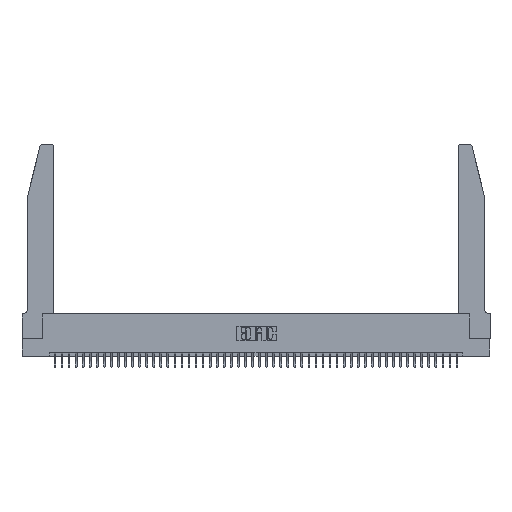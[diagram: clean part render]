
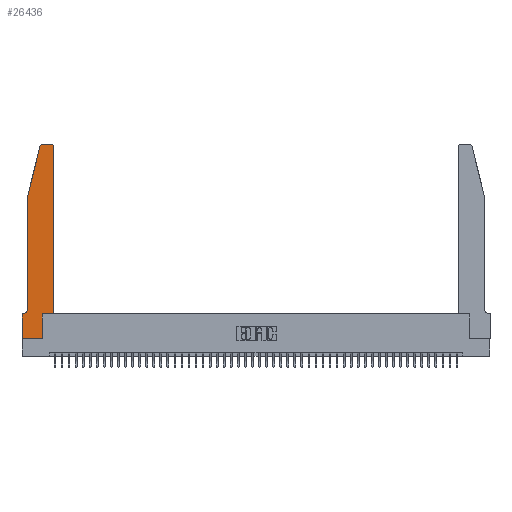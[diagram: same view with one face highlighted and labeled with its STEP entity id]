
A CAD part, top view. The second image highlights one B-rep face of the part: STEP entity #26436.
In plain terms, the highlighted planar face has unit normal (0, 0, 1).
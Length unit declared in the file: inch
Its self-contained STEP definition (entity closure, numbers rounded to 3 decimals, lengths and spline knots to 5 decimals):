
#658 = VERTEX_POINT ( 'NONE', #26307 ) ;
#1588 = VECTOR ( 'NONE', #24765, 39.37008 ) ;
#2399 = DIRECTION ( 'NONE',  ( -1., 0., 0. ) ) ;
#2454 = CARTESIAN_POINT ( 'NONE',  ( 0.0755, 0.42, 0.37 ) ) ;
#3434 = ORIENTED_EDGE ( 'NONE', *, *, #21208, .T. ) ;
#3478 = AXIS2_PLACEMENT_3D ( 'NONE', #16453, #45983, #41892 ) ;
#3490 = DIRECTION ( 'NONE',  ( 0., 0., 1. ) ) ;
#3765 = DIRECTION ( 'NONE',  ( -1., 0., 0. ) ) ;
#3785 = VERTEX_POINT ( 'NONE', #10804 ) ;
#3979 = CARTESIAN_POINT ( 'NONE',  ( 0.4205, 2.75, 0.37 ) ) ;
#4256 = CARTESIAN_POINT ( 'NONE',  ( 0., 0.35, 0.37 ) ) ;
#4416 = EDGE_CURVE ( 'NONE', #3785, #11045, #40281, .T. ) ;
#4452 = EDGE_CURVE ( 'NONE', #6735, #21793, #17524, .T. ) ;
#4508 = VECTOR ( 'NONE', #2399, 39.37008 ) ;
#4516 = VERTEX_POINT ( 'NONE', #4256 ) ;
#4940 = EDGE_CURVE ( 'NONE', #14509, #18523, #5757, .T. ) ;
#5757 = LINE ( 'NONE', #31956, #9851 ) ;
#5879 = CARTESIAN_POINT ( 'NONE',  ( 0.2865, 0.35, 0.37 ) ) ;
#6735 = VERTEX_POINT ( 'NONE', #46002 ) ;
#7153 = DIRECTION ( 'NONE',  ( 1., 0., 0. ) ) ;
#7306 = DIRECTION ( 'NONE',  ( 0., 1., 0. ) ) ;
#7971 = CARTESIAN_POINT ( 'NONE',  ( 0.2605, 2.75, 0.37 ) ) ;
#8220 = LINE ( 'NONE', #44546, #10585 ) ;
#8233 = ORIENTED_EDGE ( 'NONE', *, *, #4416, .T. ) ;
#8945 = VECTOR ( 'NONE', #47856, 39.37008 ) ;
#8959 = ORIENTED_EDGE ( 'NONE', *, *, #26096, .T. ) ;
#9250 = CARTESIAN_POINT ( 'NONE',  ( 0.4505, 2.72, 0.37 ) ) ;
#9505 = CARTESIAN_POINT ( 'NONE',  ( 0.2865, 0., 0.37 ) ) ;
#9851 = VECTOR ( 'NONE', #42897, 39.37008 ) ;
#10045 = CARTESIAN_POINT ( 'NONE',  ( 0.0755, 0.35, 0.37 ) ) ;
#10092 = CARTESIAN_POINT ( 'NONE',  ( 0., 0.35, 0.37 ) ) ;
#10585 = VECTOR ( 'NONE', #7306, 39.37008 ) ;
#10605 = CARTESIAN_POINT ( 'NONE',  ( 0.4505, 0.35, 0.37 ) ) ;
#10804 = CARTESIAN_POINT ( 'NONE',  ( 0.2865, 0.35, 0.37 ) ) ;
#11045 = VERTEX_POINT ( 'NONE', #23323 ) ;
#11275 = VERTEX_POINT ( 'NONE', #2454 ) ;
#13034 = PLANE ( 'NONE',  #36398 ) ;
#13481 = EDGE_CURVE ( 'NONE', #11045, #39683, #8220, .T. ) ;
#14509 = VERTEX_POINT ( 'NONE', #41894 ) ;
#14809 = FACE_OUTER_BOUND ( 'NONE', #20285, .T. ) ;
#14943 = ORIENTED_EDGE ( 'NONE', *, *, #48194, .T. ) ;
#15462 = EDGE_CURVE ( 'NONE', #39683, #21573, #30190, .T. ) ;
#15581 = DIRECTION ( 'NONE',  ( 1., 0., 0. ) ) ;
#15683 = ORIENTED_EDGE ( 'NONE', *, *, #47977, .T. ) ;
#16453 = CARTESIAN_POINT ( 'NONE',  ( 0.284, 2.72, 0.37 ) ) ;
#17323 = AXIS2_PLACEMENT_3D ( 'NONE', #22029, #18615, #3765 ) ;
#17524 = LINE ( 'NONE', #23445, #35010 ) ;
#17897 = EDGE_CURVE ( 'NONE', #40021, #14509, #31189, .T. ) ;
#18017 = CARTESIAN_POINT ( 'NONE',  ( 0.4205, 2.72, 0.37 ) ) ;
#18523 = VERTEX_POINT ( 'NONE', #41834 ) ;
#18615 = DIRECTION ( 'NONE',  ( 0., 0., -1. ) ) ;
#18866 = VECTOR ( 'NONE', #28699, 39.37008 ) ;
#20285 = EDGE_LOOP ( 'NONE', ( #14943, #33439, #23791, #22960, #8959, #3434, #15683, #37728, #26047, #8233, #34320, #38344 ) ) ;
#21195 = LINE ( 'NONE', #39776, #18866 ) ;
#21208 = EDGE_CURVE ( 'NONE', #658, #4516, #37759, .T. ) ;
#21354 = LINE ( 'NONE', #43546, #1588 ) ;
#21573 = VERTEX_POINT ( 'NONE', #3979 ) ;
#21793 = VERTEX_POINT ( 'NONE', #9505 ) ;
#22029 = CARTESIAN_POINT ( 'NONE',  ( 0.0055, 0.42, 0.37 ) ) ;
#22960 = ORIENTED_EDGE ( 'NONE', *, *, #34702, .T. ) ;
#23323 = CARTESIAN_POINT ( 'NONE',  ( 0.4505, 0.35, 0.37 ) ) ;
#23445 = CARTESIAN_POINT ( 'NONE',  ( 0., 0., 0.37 ) ) ;
#23791 = ORIENTED_EDGE ( 'NONE', *, *, #4940, .T. ) ;
#24765 = DIRECTION ( 'NONE',  ( 0., -1., 0. ) ) ;
#25184 = DIRECTION ( 'NONE',  ( 1., 0., 0. ) ) ;
#26047 = ORIENTED_EDGE ( 'NONE', *, *, #27686, .T. ) ;
#26096 = EDGE_CURVE ( 'NONE', #11275, #658, #46362, .T. ) ;
#26282 = VECTOR ( 'NONE', #7153, 39.37008 ) ;
#26307 = CARTESIAN_POINT ( 'NONE',  ( 0.0055, 0.35, 0.37 ) ) ;
#26436 = ADVANCED_FACE ( 'NONE', ( #14809 ), #13034, .T. ) ;
#26469 = LINE ( 'NONE', #7971, #8945 ) ;
#27686 = EDGE_CURVE ( 'NONE', #21793, #3785, #34494, .T. ) ;
#28077 = DIRECTION ( 'NONE',  ( 0., 1., 0. ) ) ;
#28194 = DIRECTION ( 'NONE',  ( 1., 0., 0. ) ) ;
#28508 = DIRECTION ( 'NONE',  ( 0., 0., 1. ) ) ;
#28699 = DIRECTION ( 'NONE',  ( 0., -1., 0. ) ) ;
#30190 = CIRCLE ( 'NONE', #39971, 0.03 ) ;
#31189 = CIRCLE ( 'NONE', #3478, 0.03 ) ;
#31956 = CARTESIAN_POINT ( 'NONE',  ( 0.0755, 2., 0.37 ) ) ;
#33439 = ORIENTED_EDGE ( 'NONE', *, *, #17897, .T. ) ;
#34320 = ORIENTED_EDGE ( 'NONE', *, *, #13481, .T. ) ;
#34494 = LINE ( 'NONE', #5879, #38031 ) ;
#34702 = EDGE_CURVE ( 'NONE', #18523, #11275, #21354, .T. ) ;
#35010 = VECTOR ( 'NONE', #15581, 39.37008 ) ;
#36398 = AXIS2_PLACEMENT_3D ( 'NONE', #10092, #28508, #28194 ) ;
#37728 = ORIENTED_EDGE ( 'NONE', *, *, #4452, .T. ) ;
#37759 = LINE ( 'NONE', #10045, #4508 ) ;
#38031 = VECTOR ( 'NONE', #28077, 39.37008 ) ;
#38344 = ORIENTED_EDGE ( 'NONE', *, *, #15462, .T. ) ;
#39683 = VERTEX_POINT ( 'NONE', #9250 ) ;
#39776 = CARTESIAN_POINT ( 'NONE',  ( 0., 0., 0.37 ) ) ;
#39971 = AXIS2_PLACEMENT_3D ( 'NONE', #18017, #3490, #25184 ) ;
#40021 = VERTEX_POINT ( 'NONE', #44326 ) ;
#40281 = LINE ( 'NONE', #10605, #26282 ) ;
#41834 = CARTESIAN_POINT ( 'NONE',  ( 0.0755, 2., 0.37 ) ) ;
#41892 = DIRECTION ( 'NONE',  ( 1., 0., 0. ) ) ;
#41894 = CARTESIAN_POINT ( 'NONE',  ( 0.25487, 2.72718, 0.37 ) ) ;
#42897 = DIRECTION ( 'NONE',  ( -0.239, -0.971, 0. ) ) ;
#43546 = CARTESIAN_POINT ( 'NONE',  ( 0.0755, 2., 0.37 ) ) ;
#44326 = CARTESIAN_POINT ( 'NONE',  ( 0.284, 2.75, 0.37 ) ) ;
#44546 = CARTESIAN_POINT ( 'NONE',  ( 0.4505, 0.35, 0.37 ) ) ;
#45983 = DIRECTION ( 'NONE',  ( 0., 0., 1. ) ) ;
#46002 = CARTESIAN_POINT ( 'NONE',  ( 0., 0., 0.37 ) ) ;
#46362 = CIRCLE ( 'NONE', #17323, 0.07 ) ;
#47856 = DIRECTION ( 'NONE',  ( -1., 0., 0. ) ) ;
#47977 = EDGE_CURVE ( 'NONE', #4516, #6735, #21195, .T. ) ;
#48194 = EDGE_CURVE ( 'NONE', #21573, #40021, #26469, .T. ) ;
